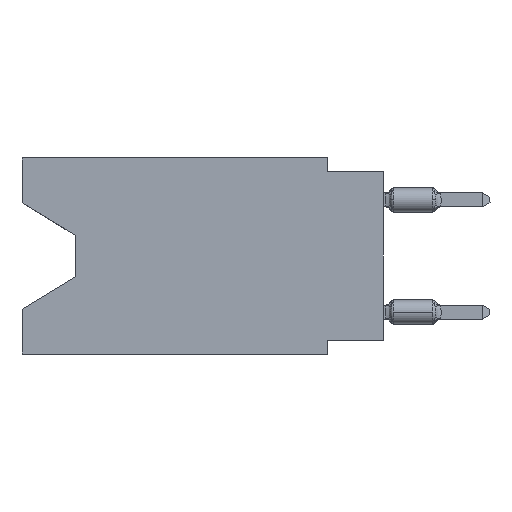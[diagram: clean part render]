
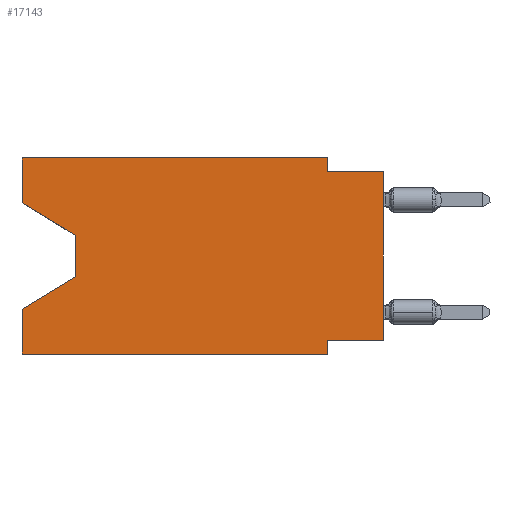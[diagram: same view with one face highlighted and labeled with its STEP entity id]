
A CAD part, left-side view. The second image highlights one B-rep face of the part: STEP entity #17143.
In plain terms, the highlighted planar face has unit normal (-1, 0, 0).
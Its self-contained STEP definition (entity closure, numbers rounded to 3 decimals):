
#80 = DIRECTION ( 'NONE',  ( 0., 0., 1. ) ) ;
#425 = CARTESIAN_POINT ( 'NONE',  ( 0., 13.97, -5.385 ) ) ;
#460 = VERTEX_POINT ( 'NONE', #9416 ) ;
#479 = VECTOR ( 'NONE', #7186, 1000. ) ;
#498 = VECTOR ( 'NONE', #12062, 1000. ) ;
#662 = ORIENTED_EDGE ( 'NONE', *, *, #6484, .T. ) ;
#886 = VECTOR ( 'NONE', #5794, 1000. ) ;
#1009 = DIRECTION ( 'NONE',  ( 0., -1., 0. ) ) ;
#1045 = LINE ( 'NONE', #8160, #10136 ) ;
#1115 = CARTESIAN_POINT ( 'NONE',  ( 0., 2.54, -0.635 ) ) ;
#1242 = CARTESIAN_POINT ( 'NONE',  ( 0., 16.383, 0. ) ) ;
#1250 = DIRECTION ( 'NONE',  ( 0., 0., -1. ) ) ;
#1407 = VECTOR ( 'NONE', #80, 1000. ) ;
#1465 = VERTEX_POINT ( 'NONE', #1115 ) ;
#1893 = CARTESIAN_POINT ( 'NONE',  ( 0., 16.383, -2.038 ) ) ;
#1948 = EDGE_CURVE ( 'NONE', #15384, #6357, #9058, .T. ) ;
#2159 = DIRECTION ( 'NONE',  ( 1., 0., 0. ) ) ;
#2296 = VECTOR ( 'NONE', #3756, 1000. ) ;
#2347 = CARTESIAN_POINT ( 'NONE',  ( 0., 13.97, -5.385 ) ) ;
#2814 = VECTOR ( 'NONE', #14298, 1000. ) ;
#3416 = ORIENTED_EDGE ( 'NONE', *, *, #1948, .F. ) ;
#3479 = PLANE ( 'NONE',  #8281 ) ;
#3756 = DIRECTION ( 'NONE',  ( 0., 0.855, -0.519 ) ) ;
#3773 = EDGE_CURVE ( 'NONE', #15384, #6935, #1045, .T. ) ;
#3837 = VECTOR ( 'NONE', #7663, 1000. ) ;
#3921 = CARTESIAN_POINT ( 'NONE',  ( 0., 2.54, -8.89 ) ) ;
#4106 = LINE ( 'NONE', #3921, #11324 ) ;
#4285 = VERTEX_POINT ( 'NONE', #11024 ) ;
#4355 = LINE ( 'NONE', #10327, #479 ) ;
#4514 = VERTEX_POINT ( 'NONE', #12135 ) ;
#4959 = LINE ( 'NONE', #6924, #7852 ) ;
#4976 = CARTESIAN_POINT ( 'NONE',  ( 0., 0., -8.255 ) ) ;
#5503 = CARTESIAN_POINT ( 'NONE',  ( 0., 2.54, -8.255 ) ) ;
#5601 = EDGE_CURVE ( 'NONE', #5905, #14381, #9449, .T. ) ;
#5794 = DIRECTION ( 'NONE',  ( 0., -1., 0. ) ) ;
#5804 = CARTESIAN_POINT ( 'NONE',  ( 0., 0., -8.255 ) ) ;
#5905 = VERTEX_POINT ( 'NONE', #425 ) ;
#6357 = VERTEX_POINT ( 'NONE', #5503 ) ;
#6458 = EDGE_CURVE ( 'NONE', #4285, #460, #14477, .T. ) ;
#6480 = DIRECTION ( 'NONE',  ( 0., -1., 0. ) ) ;
#6484 = EDGE_CURVE ( 'NONE', #14037, #5905, #4355, .T. ) ;
#6669 = EDGE_CURVE ( 'NONE', #4285, #14037, #14756, .T. ) ;
#6820 = DIRECTION ( 'NONE',  ( 0., 0., 1. ) ) ;
#6924 = CARTESIAN_POINT ( 'NONE',  ( 0., 2.54, 0. ) ) ;
#6935 = VERTEX_POINT ( 'NONE', #12939 ) ;
#7186 = DIRECTION ( 'NONE',  ( 0., 0., -1. ) ) ;
#7261 = VECTOR ( 'NONE', #6480, 1000. ) ;
#7475 = CARTESIAN_POINT ( 'NONE',  ( 0., 16.383, 0. ) ) ;
#7663 = DIRECTION ( 'NONE',  ( 0., -0.855, -0.519 ) ) ;
#7852 = VECTOR ( 'NONE', #1250, 1000. ) ;
#8160 = CARTESIAN_POINT ( 'NONE',  ( 0., 0., 0. ) ) ;
#8203 = EDGE_CURVE ( 'NONE', #14089, #1465, #4959, .T. ) ;
#8260 = ORIENTED_EDGE ( 'NONE', *, *, #3773, .T. ) ;
#8281 = AXIS2_PLACEMENT_3D ( 'NONE', #9445, #2159, #15022 ) ;
#8419 = EDGE_CURVE ( 'NONE', #10243, #4514, #17318, .T. ) ;
#8894 = ORIENTED_EDGE ( 'NONE', *, *, #6669, .T. ) ;
#9058 = LINE ( 'NONE', #4976, #498 ) ;
#9183 = CARTESIAN_POINT ( 'NONE',  ( 0., 16.383, -8.89 ) ) ;
#9416 = CARTESIAN_POINT ( 'NONE',  ( 0., 16.383, 0. ) ) ;
#9430 = EDGE_CURVE ( 'NONE', #460, #14089, #9607, .T. ) ;
#9445 = CARTESIAN_POINT ( 'NONE',  ( 0., 16.383, 0. ) ) ;
#9449 = LINE ( 'NONE', #2347, #2296 ) ;
#9607 = LINE ( 'NONE', #16979, #7261 ) ;
#9883 = DIRECTION ( 'NONE',  ( 0., 0., -1. ) ) ;
#9920 = LINE ( 'NONE', #13991, #18213 ) ;
#10136 = VECTOR ( 'NONE', #6820, 1000. ) ;
#10243 = VERTEX_POINT ( 'NONE', #9183 ) ;
#10327 = CARTESIAN_POINT ( 'NONE',  ( 0., 13.97, -3.505 ) ) ;
#11024 = CARTESIAN_POINT ( 'NONE',  ( 0., 16.383, -2.038 ) ) ;
#11324 = VECTOR ( 'NONE', #9883, 1000. ) ;
#11565 = CARTESIAN_POINT ( 'NONE',  ( 0., 2.54, 0. ) ) ;
#11691 = EDGE_LOOP ( 'NONE', ( #8894, #662, #11723, #13440, #13628, #16885, #3416, #8260, #13187, #14623, #14189, #12349 ) ) ;
#11723 = ORIENTED_EDGE ( 'NONE', *, *, #5601, .T. ) ;
#12062 = DIRECTION ( 'NONE',  ( 0., 1., 0. ) ) ;
#12135 = CARTESIAN_POINT ( 'NONE',  ( 0., 2.54, -8.89 ) ) ;
#12349 = ORIENTED_EDGE ( 'NONE', *, *, #6458, .F. ) ;
#12939 = CARTESIAN_POINT ( 'NONE',  ( 0., 0., -0.635 ) ) ;
#13187 = ORIENTED_EDGE ( 'NONE', *, *, #15820, .F. ) ;
#13440 = ORIENTED_EDGE ( 'NONE', *, *, #15648, .F. ) ;
#13628 = ORIENTED_EDGE ( 'NONE', *, *, #8419, .T. ) ;
#13991 = CARTESIAN_POINT ( 'NONE',  ( 0., 0., -0.635 ) ) ;
#14037 = VERTEX_POINT ( 'NONE', #15260 ) ;
#14089 = VERTEX_POINT ( 'NONE', #11565 ) ;
#14189 = ORIENTED_EDGE ( 'NONE', *, *, #9430, .F. ) ;
#14210 = LINE ( 'NONE', #1242, #2814 ) ;
#14298 = DIRECTION ( 'NONE',  ( 0., 0., 1. ) ) ;
#14381 = VERTEX_POINT ( 'NONE', #16654 ) ;
#14477 = LINE ( 'NONE', #7475, #1407 ) ;
#14623 = ORIENTED_EDGE ( 'NONE', *, *, #8203, .F. ) ;
#14756 = LINE ( 'NONE', #1893, #3837 ) ;
#15022 = DIRECTION ( 'NONE',  ( 0., 0., -1. ) ) ;
#15260 = CARTESIAN_POINT ( 'NONE',  ( 0., 13.97, -3.505 ) ) ;
#15384 = VERTEX_POINT ( 'NONE', #5804 ) ;
#15648 = EDGE_CURVE ( 'NONE', #10243, #14381, #14210, .T. ) ;
#15820 = EDGE_CURVE ( 'NONE', #1465, #6935, #9920, .T. ) ;
#16435 = FACE_OUTER_BOUND ( 'NONE', #11691, .T. ) ;
#16654 = CARTESIAN_POINT ( 'NONE',  ( 0., 16.383, -6.852 ) ) ;
#16885 = ORIENTED_EDGE ( 'NONE', *, *, #17708, .F. ) ;
#16979 = CARTESIAN_POINT ( 'NONE',  ( 0., 16.383, 0. ) ) ;
#17143 = ADVANCED_FACE ( 'NONE', ( #16435 ), #3479, .F. ) ;
#17230 = CARTESIAN_POINT ( 'NONE',  ( 0., 16.383, -8.89 ) ) ;
#17318 = LINE ( 'NONE', #17230, #886 ) ;
#17708 = EDGE_CURVE ( 'NONE', #6357, #4514, #4106, .T. ) ;
#18213 = VECTOR ( 'NONE', #1009, 1000. ) ;
